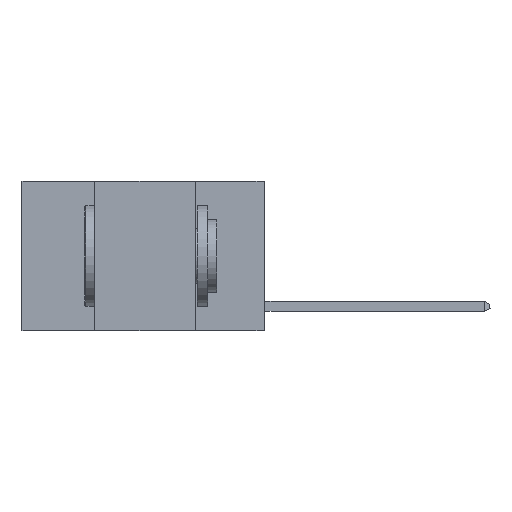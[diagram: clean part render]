
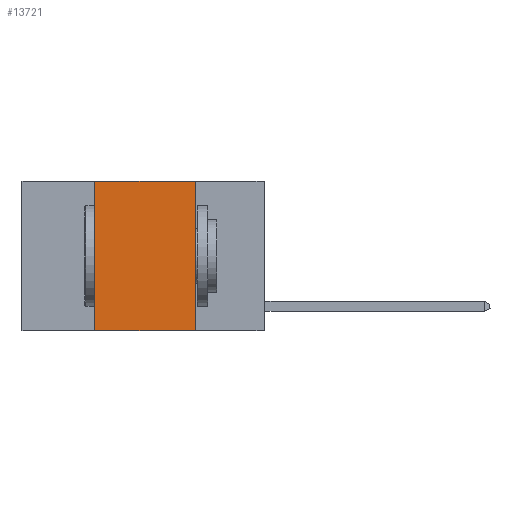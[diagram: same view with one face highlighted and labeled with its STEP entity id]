
A CAD part, left-side view. The second image highlights one B-rep face of the part: STEP entity #13721.
In plain terms, the highlighted planar face has unit normal (-1, 0, 0).
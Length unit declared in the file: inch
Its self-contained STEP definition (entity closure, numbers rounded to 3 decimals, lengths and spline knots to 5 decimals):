
#563 = DIRECTION ( 'NONE',  ( 0., 0., -1. ) ) ;
#2743 = CARTESIAN_POINT ( 'NONE',  ( 0., 0.6, -0.37 ) ) ;
#3441 = DIRECTION ( 'NONE',  ( 0., 0., 1. ) ) ;
#3568 = ORIENTED_EDGE ( 'NONE', *, *, #6571, .T. ) ;
#3855 = CARTESIAN_POINT ( 'NONE',  ( 0., 0.42, 0. ) ) ;
#4437 = PLANE ( 'NONE',  #8058 ) ;
#5171 = VECTOR ( 'NONE', #24416, 39.37008 ) ;
#6571 = EDGE_CURVE ( 'NONE', #21828, #21196, #20191, .T. ) ;
#6602 = VECTOR ( 'NONE', #3441, 39.37008 ) ;
#6841 = CARTESIAN_POINT ( 'NONE',  ( 0., 0.17, 0. ) ) ;
#6863 = VECTOR ( 'NONE', #24242, 39.37008 ) ;
#7698 = CARTESIAN_POINT ( 'NONE',  ( 0., 0.42, 0. ) ) ;
#8058 = AXIS2_PLACEMENT_3D ( 'NONE', #10340, #18142, #563 ) ;
#8874 = EDGE_LOOP ( 'NONE', ( #22649, #24129, #19036, #3568 ) ) ;
#9895 = VERTEX_POINT ( 'NONE', #3855 ) ;
#10340 = CARTESIAN_POINT ( 'NONE',  ( 0., 0.6, 0. ) ) ;
#10458 = VERTEX_POINT ( 'NONE', #21029 ) ;
#11039 = LINE ( 'NONE', #6841, #6863 ) ;
#13721 = ADVANCED_FACE ( 'NONE', ( #21998 ), #4437, .F. ) ;
#16026 = EDGE_CURVE ( 'NONE', #10458, #21196, #11039, .T. ) ;
#16633 = DIRECTION ( 'NONE',  ( 0., -1., 0. ) ) ;
#18142 = DIRECTION ( 'NONE',  ( 1., 0., 0. ) ) ;
#18438 = LINE ( 'NONE', #18694, #20476 ) ;
#18694 = CARTESIAN_POINT ( 'NONE',  ( 0., 0.6, 0. ) ) ;
#19036 = ORIENTED_EDGE ( 'NONE', *, *, #21388, .F. ) ;
#20191 = LINE ( 'NONE', #2743, #5171 ) ;
#20476 = VECTOR ( 'NONE', #16633, 39.37008 ) ;
#21029 = CARTESIAN_POINT ( 'NONE',  ( 0., 0.17, 0. ) ) ;
#21196 = VERTEX_POINT ( 'NONE', #22297 ) ;
#21233 = EDGE_CURVE ( 'NONE', #9895, #10458, #18438, .T. ) ;
#21388 = EDGE_CURVE ( 'NONE', #21828, #9895, #23043, .T. ) ;
#21828 = VERTEX_POINT ( 'NONE', #24952 ) ;
#21998 = FACE_OUTER_BOUND ( 'NONE', #8874, .T. ) ;
#22297 = CARTESIAN_POINT ( 'NONE',  ( 0., 0.17, -0.37 ) ) ;
#22649 = ORIENTED_EDGE ( 'NONE', *, *, #16026, .F. ) ;
#23043 = LINE ( 'NONE', #7698, #6602 ) ;
#24129 = ORIENTED_EDGE ( 'NONE', *, *, #21233, .F. ) ;
#24242 = DIRECTION ( 'NONE',  ( 0., 0., -1. ) ) ;
#24416 = DIRECTION ( 'NONE',  ( 0., -1., 0. ) ) ;
#24952 = CARTESIAN_POINT ( 'NONE',  ( 0., 0.42, -0.37 ) ) ;
